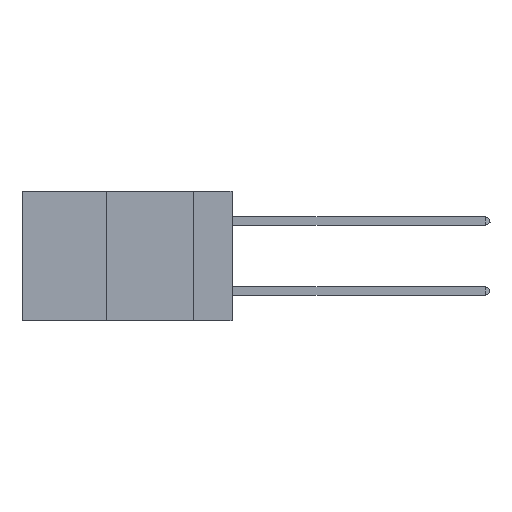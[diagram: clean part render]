
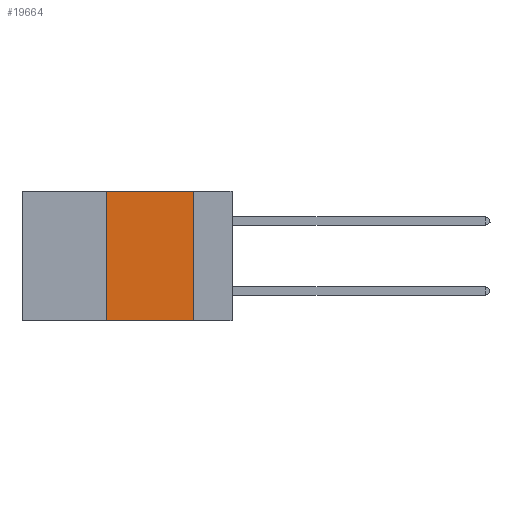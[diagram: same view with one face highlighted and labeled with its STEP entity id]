
A CAD part, left-side view. The second image highlights one B-rep face of the part: STEP entity #19664.
In plain terms, the highlighted planar face has unit normal (-1, 0, 0).
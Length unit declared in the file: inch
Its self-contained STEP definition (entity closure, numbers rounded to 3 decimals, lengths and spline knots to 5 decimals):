
#396 = ORIENTED_EDGE ( 'NONE', *, *, #3313, .F. ) ;
#1066 = CARTESIAN_POINT ( 'NONE',  ( 0., 0.11, 0. ) ) ;
#1382 = LINE ( 'NONE', #1066, #16025 ) ;
#1598 = EDGE_CURVE ( 'NONE', #2194, #10404, #7535, .T. ) ;
#1808 = EDGE_CURVE ( 'NONE', #14241, #4147, #8069, .T. ) ;
#1932 = ORIENTED_EDGE ( 'NONE', *, *, #7523, .F. ) ;
#2194 = VERTEX_POINT ( 'NONE', #13474 ) ;
#2820 = CARTESIAN_POINT ( 'NONE',  ( 0., 0.6, -0.37 ) ) ;
#3164 = CARTESIAN_POINT ( 'NONE',  ( 0., 0.36, 0. ) ) ;
#3313 = EDGE_CURVE ( 'NONE', #2194, #14241, #14645, .T. ) ;
#4003 = DIRECTION ( 'NONE',  ( 0., -1., 0. ) ) ;
#4147 = VERTEX_POINT ( 'NONE', #10770 ) ;
#4294 = DIRECTION ( 'NONE',  ( 1., 0., 0. ) ) ;
#5593 = CARTESIAN_POINT ( 'NONE',  ( 0., 0.6, 0. ) ) ;
#5678 = CARTESIAN_POINT ( 'NONE',  ( 0., 0.36, 0. ) ) ;
#7523 = EDGE_CURVE ( 'NONE', #4147, #10404, #1382, .T. ) ;
#7535 = LINE ( 'NONE', #2820, #7976 ) ;
#7976 = VECTOR ( 'NONE', #4003, 39.37008 ) ;
#8035 = EDGE_LOOP ( 'NONE', ( #1932, #17345, #396, #9297 ) ) ;
#8069 = LINE ( 'NONE', #19327, #16556 ) ;
#9297 = ORIENTED_EDGE ( 'NONE', *, *, #1598, .T. ) ;
#10404 = VERTEX_POINT ( 'NONE', #11408 ) ;
#10426 = VECTOR ( 'NONE', #12943, 39.37008 ) ;
#10770 = CARTESIAN_POINT ( 'NONE',  ( 0., 0.11, 0. ) ) ;
#11315 = DIRECTION ( 'NONE',  ( 0., -1., 0. ) ) ;
#11408 = CARTESIAN_POINT ( 'NONE',  ( 0., 0.11, -0.37 ) ) ;
#12943 = DIRECTION ( 'NONE',  ( 0., 0., 1. ) ) ;
#13369 = AXIS2_PLACEMENT_3D ( 'NONE', #5593, #4294, #18785 ) ;
#13474 = CARTESIAN_POINT ( 'NONE',  ( 0., 0.36, -0.37 ) ) ;
#14241 = VERTEX_POINT ( 'NONE', #5678 ) ;
#14645 = LINE ( 'NONE', #3164, #10426 ) ;
#16025 = VECTOR ( 'NONE', #17676, 39.37008 ) ;
#16556 = VECTOR ( 'NONE', #11315, 39.37008 ) ;
#17197 = FACE_OUTER_BOUND ( 'NONE', #8035, .T. ) ;
#17345 = ORIENTED_EDGE ( 'NONE', *, *, #1808, .F. ) ;
#17676 = DIRECTION ( 'NONE',  ( 0., 0., -1. ) ) ;
#18785 = DIRECTION ( 'NONE',  ( 0., 0., -1. ) ) ;
#19327 = CARTESIAN_POINT ( 'NONE',  ( 0., 0.6, 0. ) ) ;
#19664 = ADVANCED_FACE ( 'NONE', ( #17197 ), #20305, .F. ) ;
#20305 = PLANE ( 'NONE',  #13369 ) ;
